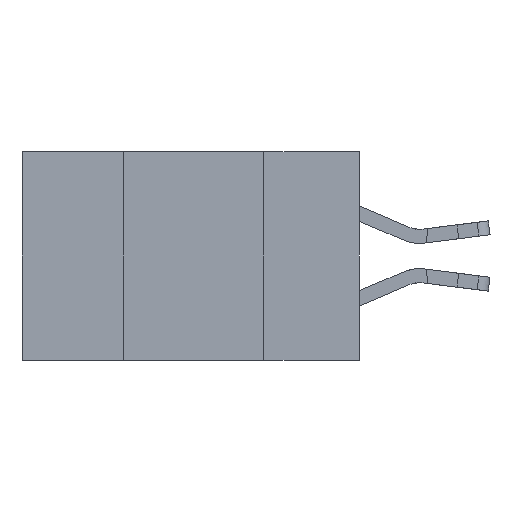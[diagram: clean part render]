
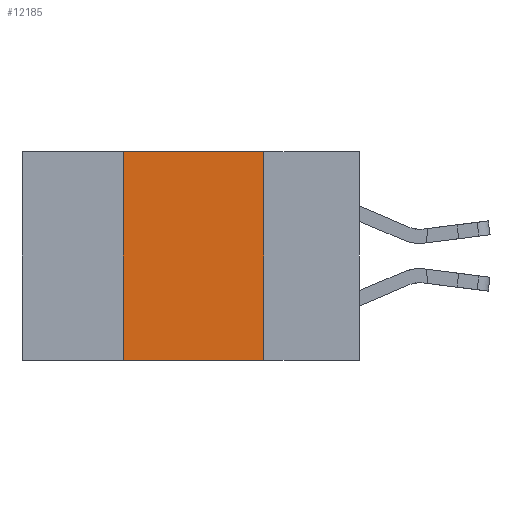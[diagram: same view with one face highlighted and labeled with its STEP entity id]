
A CAD part, left-side view. The second image highlights one B-rep face of the part: STEP entity #12185.
In plain terms, the highlighted planar face has unit normal (-1, 0, 0).
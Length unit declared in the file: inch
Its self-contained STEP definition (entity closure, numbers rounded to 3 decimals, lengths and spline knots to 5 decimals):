
#959 = PLANE ( 'NONE',  #1237 ) ;
#1074 = EDGE_CURVE ( 'NONE', #5857, #10076, #8232, .T. ) ;
#1237 = AXIS2_PLACEMENT_3D ( 'NONE', #7805, #3703, #8842 ) ;
#1632 = CARTESIAN_POINT ( 'NONE',  ( 0., 0.6, -0.37 ) ) ;
#3022 = CARTESIAN_POINT ( 'NONE',  ( 0., 0.42, 0. ) ) ;
#3571 = VERTEX_POINT ( 'NONE', #11506 ) ;
#3585 = ORIENTED_EDGE ( 'NONE', *, *, #1074, .T. ) ;
#3703 = DIRECTION ( 'NONE',  ( 1., 0., 0. ) ) ;
#5446 = DIRECTION ( 'NONE',  ( 0., -1., 0. ) ) ;
#5675 = DIRECTION ( 'NONE',  ( 0., 0., 1. ) ) ;
#5771 = CARTESIAN_POINT ( 'NONE',  ( 0., 0.17, 0. ) ) ;
#5857 = VERTEX_POINT ( 'NONE', #11477 ) ;
#6764 = EDGE_LOOP ( 'NONE', ( #11775, #8334, #15140, #3585 ) ) ;
#7287 = LINE ( 'NONE', #5771, #11941 ) ;
#7805 = CARTESIAN_POINT ( 'NONE',  ( 0., 0.6, 0. ) ) ;
#8058 = LINE ( 'NONE', #3022, #11068 ) ;
#8097 = EDGE_CURVE ( 'NONE', #5857, #13838, #8058, .T. ) ;
#8232 = LINE ( 'NONE', #1632, #9248 ) ;
#8334 = ORIENTED_EDGE ( 'NONE', *, *, #14115, .F. ) ;
#8808 = CARTESIAN_POINT ( 'NONE',  ( 0., 0.17, -0.37 ) ) ;
#8842 = DIRECTION ( 'NONE',  ( 0., 0., -1. ) ) ;
#9248 = VECTOR ( 'NONE', #9540, 39.37008 ) ;
#9540 = DIRECTION ( 'NONE',  ( 0., -1., 0. ) ) ;
#9675 = CARTESIAN_POINT ( 'NONE',  ( 0., 0.42, 0. ) ) ;
#10076 = VERTEX_POINT ( 'NONE', #8808 ) ;
#10422 = LINE ( 'NONE', #11702, #14093 ) ;
#10995 = DIRECTION ( 'NONE',  ( 0., 0., -1. ) ) ;
#11068 = VECTOR ( 'NONE', #5675, 39.37008 ) ;
#11477 = CARTESIAN_POINT ( 'NONE',  ( 0., 0.42, -0.37 ) ) ;
#11506 = CARTESIAN_POINT ( 'NONE',  ( 0., 0.17, 0. ) ) ;
#11702 = CARTESIAN_POINT ( 'NONE',  ( 0., 0.6, 0. ) ) ;
#11775 = ORIENTED_EDGE ( 'NONE', *, *, #12947, .F. ) ;
#11941 = VECTOR ( 'NONE', #10995, 39.37008 ) ;
#12185 = ADVANCED_FACE ( 'NONE', ( #13046 ), #959, .F. ) ;
#12947 = EDGE_CURVE ( 'NONE', #3571, #10076, #7287, .T. ) ;
#13046 = FACE_OUTER_BOUND ( 'NONE', #6764, .T. ) ;
#13838 = VERTEX_POINT ( 'NONE', #9675 ) ;
#14093 = VECTOR ( 'NONE', #5446, 39.37008 ) ;
#14115 = EDGE_CURVE ( 'NONE', #13838, #3571, #10422, .T. ) ;
#15140 = ORIENTED_EDGE ( 'NONE', *, *, #8097, .F. ) ;
